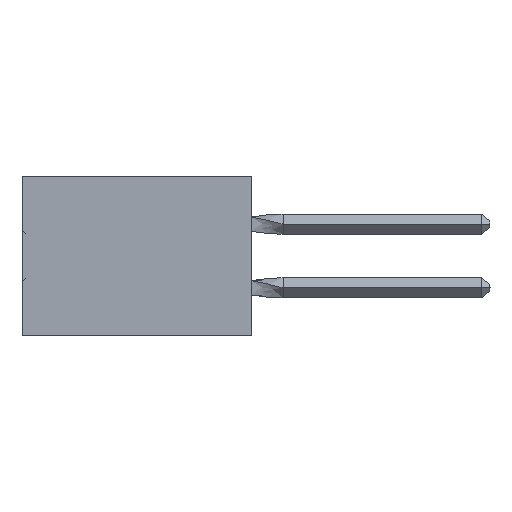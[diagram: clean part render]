
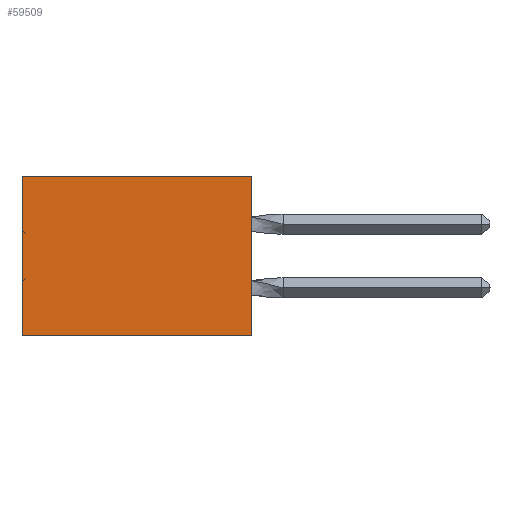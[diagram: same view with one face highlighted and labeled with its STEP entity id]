
A CAD part, left-side view. The second image highlights one B-rep face of the part: STEP entity #59509.
In plain terms, the highlighted planar face has unit normal (-1, 0, 0).
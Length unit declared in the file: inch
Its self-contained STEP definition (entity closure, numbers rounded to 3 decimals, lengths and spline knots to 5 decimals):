
#178 = DIRECTION ( 'NONE',  ( 0., 1., 0. ) ) ;
#817 = ORIENTED_EDGE ( 'NONE', *, *, #45906, .F. ) ;
#2016 = ORIENTED_EDGE ( 'NONE', *, *, #34622, .T. ) ;
#2884 = EDGE_LOOP ( 'NONE', ( #53185, #817, #41519, #2016 ) ) ;
#3048 = CARTESIAN_POINT ( 'NONE',  ( 0.305, 0.72, -0.5 ) ) ;
#7387 = VECTOR ( 'NONE', #60077, 39.37008 ) ;
#8170 = PLANE ( 'NONE',  #21703 ) ;
#9427 = VERTEX_POINT ( 'NONE', #56816 ) ;
#10681 = CARTESIAN_POINT ( 'NONE',  ( 0.305, 0., -0.5 ) ) ;
#11030 = LINE ( 'NONE', #39432, #15356 ) ;
#15356 = VECTOR ( 'NONE', #52879, 39.37008 ) ;
#16218 = VECTOR ( 'NONE', #21822, 39.37008 ) ;
#18288 = FACE_OUTER_BOUND ( 'NONE', #2884, .T. ) ;
#21703 = AXIS2_PLACEMENT_3D ( 'NONE', #54561, #53979, #26923 ) ;
#21822 = DIRECTION ( 'NONE',  ( 0., 0., -1. ) ) ;
#25385 = CARTESIAN_POINT ( 'NONE',  ( 0.305, 0.72, -0.5 ) ) ;
#26923 = DIRECTION ( 'NONE',  ( 0., 0., -1. ) ) ;
#32166 = LINE ( 'NONE', #3048, #16218 ) ;
#33986 = EDGE_CURVE ( 'NONE', #9427, #55465, #32166, .T. ) ;
#34622 = EDGE_CURVE ( 'NONE', #43240, #9427, #44521, .T. ) ;
#34869 = EDGE_CURVE ( 'NONE', #43240, #52653, #11030, .T. ) ;
#36436 = CARTESIAN_POINT ( 'NONE',  ( 0.305, 0., 0. ) ) ;
#39432 = CARTESIAN_POINT ( 'NONE',  ( 0.305, 0., -0.5 ) ) ;
#41519 = ORIENTED_EDGE ( 'NONE', *, *, #34869, .F. ) ;
#43240 = VERTEX_POINT ( 'NONE', #36436 ) ;
#44521 = LINE ( 'NONE', #46176, #48097 ) ;
#45906 = EDGE_CURVE ( 'NONE', #52653, #55465, #54056, .T. ) ;
#46176 = CARTESIAN_POINT ( 'NONE',  ( 0.305, 0., 0. ) ) ;
#48097 = VECTOR ( 'NONE', #178, 39.37008 ) ;
#50746 = CARTESIAN_POINT ( 'NONE',  ( 0.305, 0., -0.5 ) ) ;
#52653 = VERTEX_POINT ( 'NONE', #10681 ) ;
#52879 = DIRECTION ( 'NONE',  ( 0., 0., -1. ) ) ;
#53185 = ORIENTED_EDGE ( 'NONE', *, *, #33986, .T. ) ;
#53979 = DIRECTION ( 'NONE',  ( 1., 0., 0. ) ) ;
#54056 = LINE ( 'NONE', #50746, #7387 ) ;
#54561 = CARTESIAN_POINT ( 'NONE',  ( 0.305, 0., -0.5 ) ) ;
#55465 = VERTEX_POINT ( 'NONE', #25385 ) ;
#56816 = CARTESIAN_POINT ( 'NONE',  ( 0.305, 0.72, 0. ) ) ;
#59509 = ADVANCED_FACE ( 'NONE', ( #18288 ), #8170, .F. ) ;
#60077 = DIRECTION ( 'NONE',  ( 0., 1., 0. ) ) ;
